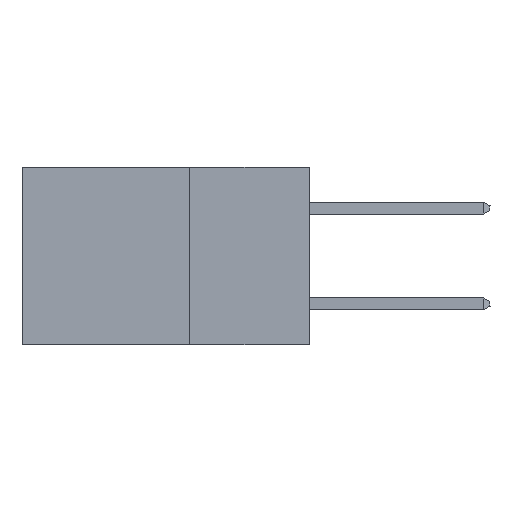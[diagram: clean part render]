
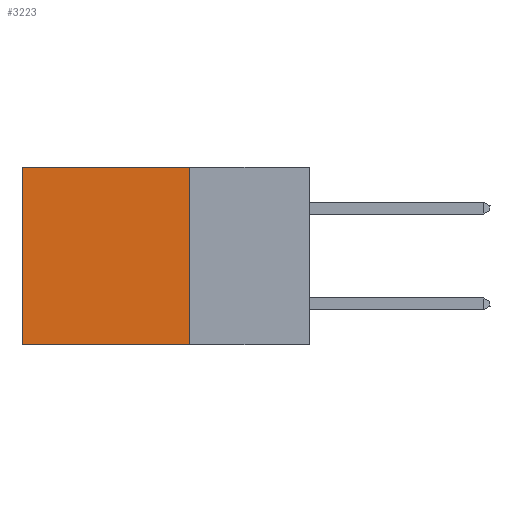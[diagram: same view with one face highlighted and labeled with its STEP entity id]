
A CAD part, left-side view. The second image highlights one B-rep face of the part: STEP entity #3223.
In plain terms, the highlighted planar face has unit normal (-1, 0, 0).
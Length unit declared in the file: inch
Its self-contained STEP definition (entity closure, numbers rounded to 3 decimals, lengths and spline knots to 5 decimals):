
#960 = VERTEX_POINT ( 'NONE', #9354 ) ;
#1256 = CARTESIAN_POINT ( 'NONE',  ( 0.2875, 0.6, 0. ) ) ;
#2390 = EDGE_CURVE ( 'NONE', #960, #19964, #3602, .T. ) ;
#2563 = CARTESIAN_POINT ( 'NONE',  ( 0.2875, 0.25, -0.37 ) ) ;
#2803 = ORIENTED_EDGE ( 'NONE', *, *, #3245, .F. ) ;
#3223 = ADVANCED_FACE ( 'NONE', ( #6387 ), #6114, .F. ) ;
#3245 = EDGE_CURVE ( 'NONE', #19964, #21135, #5830, .T. ) ;
#3498 = LINE ( 'NONE', #1256, #16899 ) ;
#3602 = LINE ( 'NONE', #3942, #17009 ) ;
#3942 = CARTESIAN_POINT ( 'NONE',  ( 0.2875, 0.25, 0. ) ) ;
#4098 = EDGE_CURVE ( 'NONE', #960, #5656, #20127, .T. ) ;
#5656 = VERTEX_POINT ( 'NONE', #7536 ) ;
#5830 = LINE ( 'NONE', #2563, #9944 ) ;
#6114 = PLANE ( 'NONE',  #8425 ) ;
#6387 = FACE_OUTER_BOUND ( 'NONE', #8397, .T. ) ;
#6570 = CARTESIAN_POINT ( 'NONE',  ( 0.2875, 0.25, 0. ) ) ;
#7536 = CARTESIAN_POINT ( 'NONE',  ( 0.2875, 0.6, 0. ) ) ;
#7889 = DIRECTION ( 'NONE',  ( 0., 0., -1. ) ) ;
#8221 = CARTESIAN_POINT ( 'NONE',  ( 0.2875, 0.25, -0.37 ) ) ;
#8397 = EDGE_LOOP ( 'NONE', ( #13118, #2803, #22423, #20424 ) ) ;
#8425 = AXIS2_PLACEMENT_3D ( 'NONE', #11279, #18247, #7889 ) ;
#9354 = CARTESIAN_POINT ( 'NONE',  ( 0.2875, 0.25, 0. ) ) ;
#9944 = VECTOR ( 'NONE', #16581, 39.37008 ) ;
#11009 = VECTOR ( 'NONE', #18656, 39.37008 ) ;
#11279 = CARTESIAN_POINT ( 'NONE',  ( 0.2875, 0.25, 0. ) ) ;
#11901 = DIRECTION ( 'NONE',  ( 0., 0., -1. ) ) ;
#13118 = ORIENTED_EDGE ( 'NONE', *, *, #13464, .T. ) ;
#13464 = EDGE_CURVE ( 'NONE', #5656, #21135, #3498, .T. ) ;
#16170 = DIRECTION ( 'NONE',  ( 0., 0., -1. ) ) ;
#16581 = DIRECTION ( 'NONE',  ( 0., 1., 0. ) ) ;
#16899 = VECTOR ( 'NONE', #11901, 39.37008 ) ;
#17009 = VECTOR ( 'NONE', #16170, 39.37008 ) ;
#18247 = DIRECTION ( 'NONE',  ( 1., 0., 0. ) ) ;
#18656 = DIRECTION ( 'NONE',  ( 0., 1., 0. ) ) ;
#19964 = VERTEX_POINT ( 'NONE', #8221 ) ;
#20127 = LINE ( 'NONE', #6570, #11009 ) ;
#20424 = ORIENTED_EDGE ( 'NONE', *, *, #4098, .T. ) ;
#20821 = CARTESIAN_POINT ( 'NONE',  ( 0.2875, 0.6, -0.37 ) ) ;
#21135 = VERTEX_POINT ( 'NONE', #20821 ) ;
#22423 = ORIENTED_EDGE ( 'NONE', *, *, #2390, .F. ) ;
